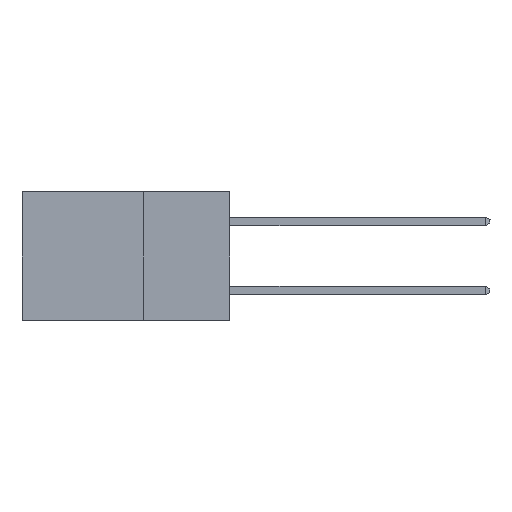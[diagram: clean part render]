
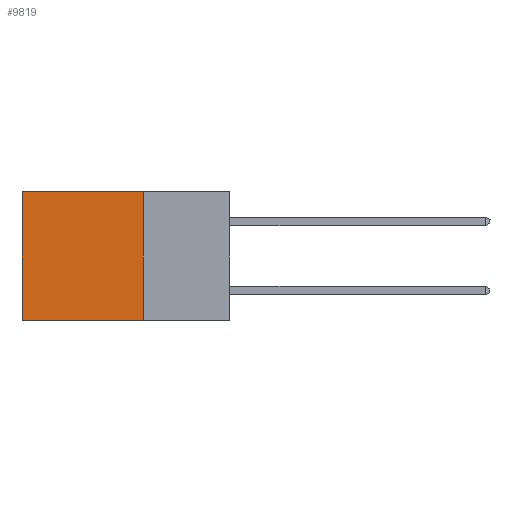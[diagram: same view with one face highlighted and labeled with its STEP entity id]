
A CAD part, left-side view. The second image highlights one B-rep face of the part: STEP entity #9819.
In plain terms, the highlighted planar face has unit normal (-1, 0, 0).
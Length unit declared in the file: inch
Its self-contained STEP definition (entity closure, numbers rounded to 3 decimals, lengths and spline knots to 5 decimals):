
#249 = CARTESIAN_POINT ( 'NONE',  ( 0.2615, 0.25, 0. ) ) ;
#513 = CARTESIAN_POINT ( 'NONE',  ( 0.2615, 0.25, -0.37 ) ) ;
#853 = DIRECTION ( 'NONE',  ( 0., 0., -1. ) ) ;
#1125 = DIRECTION ( 'NONE',  ( 0., 0., -1. ) ) ;
#2080 = VECTOR ( 'NONE', #14064, 39.37008 ) ;
#2191 = AXIS2_PLACEMENT_3D ( 'NONE', #13380, #8626, #853 ) ;
#2834 = LINE ( 'NONE', #14192, #14520 ) ;
#2845 = CARTESIAN_POINT ( 'NONE',  ( 0.2615, 0.25, -0.37 ) ) ;
#3007 = EDGE_LOOP ( 'NONE', ( #9991, #14560, #14287, #8289 ) ) ;
#3101 = DIRECTION ( 'NONE',  ( 0., 0., -1. ) ) ;
#3672 = EDGE_CURVE ( 'NONE', #5719, #11927, #4138, .T. ) ;
#4138 = LINE ( 'NONE', #7542, #12928 ) ;
#5359 = PLANE ( 'NONE',  #2191 ) ;
#5719 = VERTEX_POINT ( 'NONE', #249 ) ;
#6054 = VERTEX_POINT ( 'NONE', #6753 ) ;
#6100 = VECTOR ( 'NONE', #1125, 39.37008 ) ;
#6386 = CARTESIAN_POINT ( 'NONE',  ( 0.2615, 0.6, -0.37 ) ) ;
#6753 = CARTESIAN_POINT ( 'NONE',  ( 0.2615, 0.6, 0. ) ) ;
#7542 = CARTESIAN_POINT ( 'NONE',  ( 0.2615, 0.25, -0.37 ) ) ;
#8289 = ORIENTED_EDGE ( 'NONE', *, *, #9489, .T. ) ;
#8626 = DIRECTION ( 'NONE',  ( 1., 0., 0. ) ) ;
#8734 = LINE ( 'NONE', #14619, #6100 ) ;
#9002 = VERTEX_POINT ( 'NONE', #6386 ) ;
#9489 = EDGE_CURVE ( 'NONE', #5719, #6054, #2834, .T. ) ;
#9819 = ADVANCED_FACE ( 'NONE', ( #10613 ), #5359, .F. ) ;
#9991 = ORIENTED_EDGE ( 'NONE', *, *, #14346, .T. ) ;
#10613 = FACE_OUTER_BOUND ( 'NONE', #3007, .T. ) ;
#11416 = EDGE_CURVE ( 'NONE', #11927, #9002, #13918, .T. ) ;
#11927 = VERTEX_POINT ( 'NONE', #513 ) ;
#11973 = DIRECTION ( 'NONE',  ( 0., 1., 0. ) ) ;
#12928 = VECTOR ( 'NONE', #3101, 39.37008 ) ;
#13380 = CARTESIAN_POINT ( 'NONE',  ( 0.2615, 0.25, -0.37 ) ) ;
#13918 = LINE ( 'NONE', #2845, #2080 ) ;
#14064 = DIRECTION ( 'NONE',  ( 0., 1., 0. ) ) ;
#14192 = CARTESIAN_POINT ( 'NONE',  ( 0.2615, 0.25, 0. ) ) ;
#14287 = ORIENTED_EDGE ( 'NONE', *, *, #3672, .F. ) ;
#14346 = EDGE_CURVE ( 'NONE', #6054, #9002, #8734, .T. ) ;
#14520 = VECTOR ( 'NONE', #11973, 39.37008 ) ;
#14560 = ORIENTED_EDGE ( 'NONE', *, *, #11416, .F. ) ;
#14619 = CARTESIAN_POINT ( 'NONE',  ( 0.2615, 0.6, -0.37 ) ) ;
